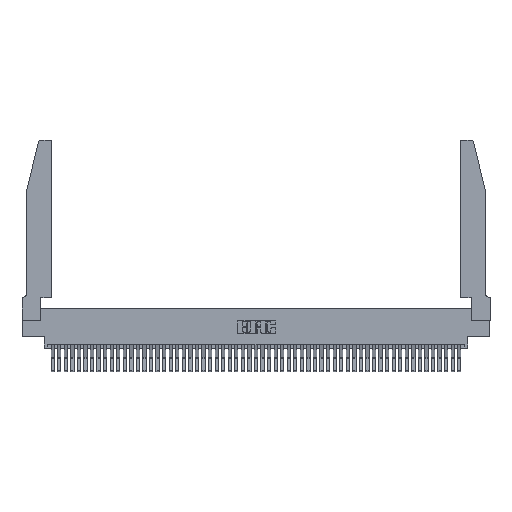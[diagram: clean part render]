
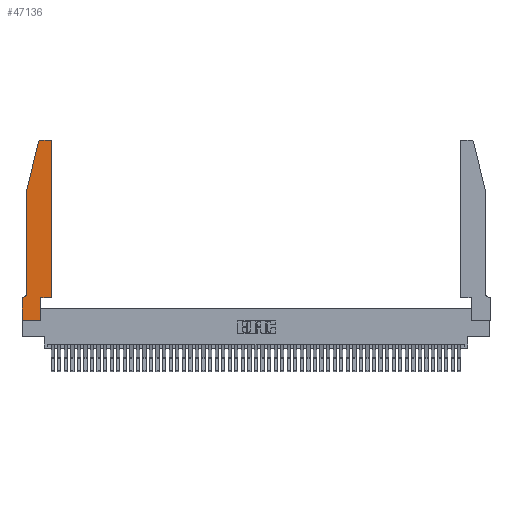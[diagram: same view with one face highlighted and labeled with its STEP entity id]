
A CAD part, top view. The second image highlights one B-rep face of the part: STEP entity #47136.
In plain terms, the highlighted planar face has unit normal (0, 0, 1).
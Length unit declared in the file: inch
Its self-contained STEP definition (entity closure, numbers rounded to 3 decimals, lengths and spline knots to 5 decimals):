
#366 = VERTEX_POINT ( 'NONE', #22037 ) ;
#576 = EDGE_CURVE ( 'NONE', #25465, #22878, #44019, .T. ) ;
#1135 = CARTESIAN_POINT ( 'NONE',  ( 0.284, 2.72, 0.37 ) ) ;
#2514 = CARTESIAN_POINT ( 'NONE',  ( 0.4505, 0.35, 0.37 ) ) ;
#2733 = ORIENTED_EDGE ( 'NONE', *, *, #31562, .T. ) ;
#2984 = CARTESIAN_POINT ( 'NONE',  ( 0.0755, 2., 0.37 ) ) ;
#3062 = DIRECTION ( 'NONE',  ( 0., 0., -1. ) ) ;
#3526 = CARTESIAN_POINT ( 'NONE',  ( 0., 0., 0.37 ) ) ;
#3726 = DIRECTION ( 'NONE',  ( 1., 0., 0. ) ) ;
#3866 = ORIENTED_EDGE ( 'NONE', *, *, #28740, .T. ) ;
#4680 = CARTESIAN_POINT ( 'NONE',  ( 0.2865, 0., 0.37 ) ) ;
#4715 = EDGE_LOOP ( 'NONE', ( #38875, #14616, #37971, #31926, #16359, #17977, #21294, #2733, #43229, #3866, #4978, #11433 ) ) ;
#4978 = ORIENTED_EDGE ( 'NONE', *, *, #38837, .T. ) ;
#5257 = DIRECTION ( 'NONE',  ( 1., 0., 0. ) ) ;
#6131 = CARTESIAN_POINT ( 'NONE',  ( 0.0755, 2., 0.37 ) ) ;
#6942 = CIRCLE ( 'NONE', #12541, 0.07 ) ;
#7370 = EDGE_CURVE ( 'NONE', #25886, #43570, #14643, .T. ) ;
#7718 = DIRECTION ( 'NONE',  ( 0., 1., 0. ) ) ;
#7939 = DIRECTION ( 'NONE',  ( -1., 0., 0. ) ) ;
#8092 = CARTESIAN_POINT ( 'NONE',  ( 0., 0.35, 0.37 ) ) ;
#8425 = DIRECTION ( 'NONE',  ( 0., -1., 0. ) ) ;
#8459 = VERTEX_POINT ( 'NONE', #22975 ) ;
#8475 = EDGE_CURVE ( 'NONE', #22878, #50640, #6942, .T. ) ;
#10042 = LINE ( 'NONE', #2514, #20710 ) ;
#11019 = DIRECTION ( 'NONE',  ( 0., -1., 0. ) ) ;
#11200 = FACE_OUTER_BOUND ( 'NONE', #4715, .T. ) ;
#11433 = ORIENTED_EDGE ( 'NONE', *, *, #18001, .T. ) ;
#11448 = DIRECTION ( 'NONE',  ( 1., 0., 0. ) ) ;
#11584 = LINE ( 'NONE', #51332, #20977 ) ;
#11618 = LINE ( 'NONE', #36181, #40824 ) ;
#11827 = VERTEX_POINT ( 'NONE', #26515 ) ;
#12148 = DIRECTION ( 'NONE',  ( 1., 0., 0. ) ) ;
#12541 = AXIS2_PLACEMENT_3D ( 'NONE', #27162, #3062, #31143 ) ;
#13393 = VECTOR ( 'NONE', #7718, 39.37008 ) ;
#14616 = ORIENTED_EDGE ( 'NONE', *, *, #18747, .T. ) ;
#14643 = LINE ( 'NONE', #15826, #13393 ) ;
#14647 = LINE ( 'NONE', #31863, #26505 ) ;
#15316 = CARTESIAN_POINT ( 'NONE',  ( 0.4505, 0.35, 0.37 ) ) ;
#15521 = LINE ( 'NONE', #38647, #28620 ) ;
#15678 = VERTEX_POINT ( 'NONE', #49420 ) ;
#15826 = CARTESIAN_POINT ( 'NONE',  ( 0.2865, 0.35, 0.37 ) ) ;
#16193 = VECTOR ( 'NONE', #11448, 39.37008 ) ;
#16359 = ORIENTED_EDGE ( 'NONE', *, *, #8475, .T. ) ;
#17009 = DIRECTION ( 'NONE',  ( 0., 0., 1. ) ) ;
#17276 = VERTEX_POINT ( 'NONE', #24381 ) ;
#17977 = ORIENTED_EDGE ( 'NONE', *, *, #41471, .T. ) ;
#18001 = EDGE_CURVE ( 'NONE', #17276, #15678, #46064, .T. ) ;
#18747 = EDGE_CURVE ( 'NONE', #11827, #37940, #47869, .T. ) ;
#18783 = DIRECTION ( 'NONE',  ( 0., 1., 0. ) ) ;
#19467 = AXIS2_PLACEMENT_3D ( 'NONE', #8092, #35989, #12148 ) ;
#20026 = CARTESIAN_POINT ( 'NONE',  ( 0.2865, 0.35, 0.37 ) ) ;
#20347 = CARTESIAN_POINT ( 'NONE',  ( 0., 0., 0.37 ) ) ;
#20388 = DIRECTION ( 'NONE',  ( -0.239, -0.971, 0. ) ) ;
#20710 = VECTOR ( 'NONE', #18783, 39.37008 ) ;
#20977 = VECTOR ( 'NONE', #3726, 39.37008 ) ;
#21294 = ORIENTED_EDGE ( 'NONE', *, *, #28901, .T. ) ;
#21480 = CARTESIAN_POINT ( 'NONE',  ( 0.25487, 2.72718, 0.37 ) ) ;
#22037 = CARTESIAN_POINT ( 'NONE',  ( 0.4505, 0.35, 0.37 ) ) ;
#22362 = CARTESIAN_POINT ( 'NONE',  ( 0.0055, 0.35, 0.37 ) ) ;
#22878 = VERTEX_POINT ( 'NONE', #40115 ) ;
#22975 = CARTESIAN_POINT ( 'NONE',  ( 0., 0.35, 0.37 ) ) ;
#24381 = CARTESIAN_POINT ( 'NONE',  ( 0.4505, 2.72, 0.37 ) ) ;
#25465 = VERTEX_POINT ( 'NONE', #6131 ) ;
#25886 = VERTEX_POINT ( 'NONE', #4680 ) ;
#26505 = VECTOR ( 'NONE', #7939, 39.37008 ) ;
#26515 = CARTESIAN_POINT ( 'NONE',  ( 0.284, 2.75, 0.37 ) ) ;
#27162 = CARTESIAN_POINT ( 'NONE',  ( 0.0055, 0.42, 0.37 ) ) ;
#28620 = VECTOR ( 'NONE', #42583, 39.37008 ) ;
#28740 = EDGE_CURVE ( 'NONE', #43570, #366, #46512, .T. ) ;
#28901 = EDGE_CURVE ( 'NONE', #8459, #33492, #50786, .T. ) ;
#29011 = AXIS2_PLACEMENT_3D ( 'NONE', #1135, #29278, #5257 ) ;
#29278 = DIRECTION ( 'NONE',  ( 0., 0., 1. ) ) ;
#31143 = DIRECTION ( 'NONE',  ( -1., 0., 0. ) ) ;
#31562 = EDGE_CURVE ( 'NONE', #33492, #25886, #11584, .T. ) ;
#31863 = CARTESIAN_POINT ( 'NONE',  ( 0.2605, 2.75, 0.37 ) ) ;
#31926 = ORIENTED_EDGE ( 'NONE', *, *, #576, .T. ) ;
#32138 = EDGE_CURVE ( 'NONE', #15678, #11827, #14647, .T. ) ;
#33492 = VERTEX_POINT ( 'NONE', #3526 ) ;
#35989 = DIRECTION ( 'NONE',  ( 0., 0., 1. ) ) ;
#36181 = CARTESIAN_POINT ( 'NONE',  ( 0.0755, 2., 0.37 ) ) ;
#37940 = VERTEX_POINT ( 'NONE', #21480 ) ;
#37971 = ORIENTED_EDGE ( 'NONE', *, *, #49625, .T. ) ;
#38647 = CARTESIAN_POINT ( 'NONE',  ( 0.0755, 0.35, 0.37 ) ) ;
#38837 = EDGE_CURVE ( 'NONE', #366, #17276, #10042, .T. ) ;
#38875 = ORIENTED_EDGE ( 'NONE', *, *, #32138, .T. ) ;
#40115 = CARTESIAN_POINT ( 'NONE',  ( 0.0755, 0.42, 0.37 ) ) ;
#40753 = CARTESIAN_POINT ( 'NONE',  ( 0.4205, 2.72, 0.37 ) ) ;
#40824 = VECTOR ( 'NONE', #20388, 39.37008 ) ;
#41471 = EDGE_CURVE ( 'NONE', #50640, #8459, #15521, .T. ) ;
#42583 = DIRECTION ( 'NONE',  ( -1., 0., 0. ) ) ;
#42784 = VECTOR ( 'NONE', #11019, 39.37008 ) ;
#43229 = ORIENTED_EDGE ( 'NONE', *, *, #7370, .T. ) ;
#43570 = VERTEX_POINT ( 'NONE', #20026 ) ;
#44019 = LINE ( 'NONE', #2984, #42784 ) ;
#44670 = DIRECTION ( 'NONE',  ( 1., 0., 0. ) ) ;
#46064 = CIRCLE ( 'NONE', #51245, 0.03 ) ;
#46512 = LINE ( 'NONE', #15316, #16193 ) ;
#47136 = ADVANCED_FACE ( 'NONE', ( #11200 ), #47666, .T. ) ;
#47666 = PLANE ( 'NONE',  #19467 ) ;
#47869 = CIRCLE ( 'NONE', #29011, 0.03 ) ;
#49420 = CARTESIAN_POINT ( 'NONE',  ( 0.4205, 2.75, 0.37 ) ) ;
#49553 = VECTOR ( 'NONE', #8425, 39.37008 ) ;
#49625 = EDGE_CURVE ( 'NONE', #37940, #25465, #11618, .T. ) ;
#50640 = VERTEX_POINT ( 'NONE', #22362 ) ;
#50786 = LINE ( 'NONE', #20347, #49553 ) ;
#51245 = AXIS2_PLACEMENT_3D ( 'NONE', #40753, #17009, #44670 ) ;
#51332 = CARTESIAN_POINT ( 'NONE',  ( 0., 0., 0.37 ) ) ;
